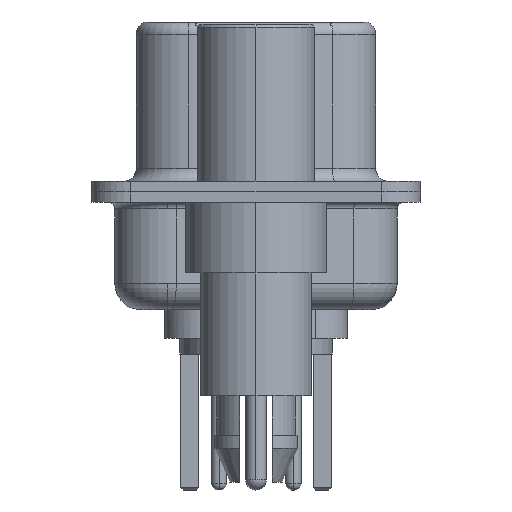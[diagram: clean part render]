
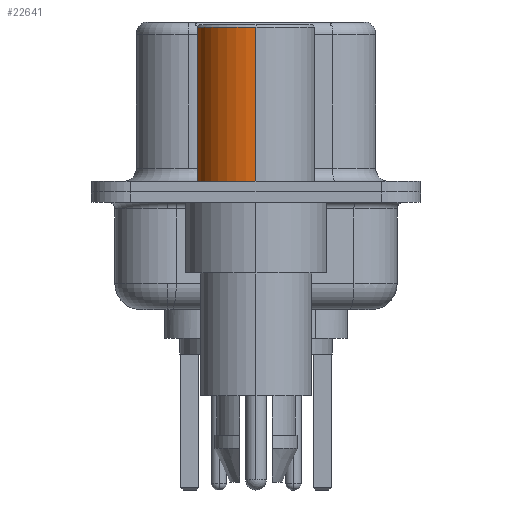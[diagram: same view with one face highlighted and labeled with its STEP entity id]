
A CAD part, left-side view. The second image highlights one B-rep face of the part: STEP entity #22641.
In plain terms, the highlighted cylindrical face has radius 2.25 mm (diameter 4.5 mm), a partial arc.
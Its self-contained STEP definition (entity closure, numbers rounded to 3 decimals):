
#1869 = CARTESIAN_POINT ( 'NONE',  ( -2.25, 0., 0.581 ) ) ;
#3920 = DIRECTION ( 'NONE',  ( 0., 0., 1. ) ) ;
#3991 = LINE ( 'NONE', #20958, #14371 ) ;
#4798 = CIRCLE ( 'NONE', #10712, 2.25 ) ;
#5557 = DIRECTION ( 'NONE',  ( 0., 0., 1. ) ) ;
#6563 = DIRECTION ( 'NONE',  ( 0., 0., 1. ) ) ;
#7270 = DIRECTION ( 'NONE',  ( 0., 0., 1. ) ) ;
#7772 = CARTESIAN_POINT ( 'NONE',  ( -2.25, 0., 0.4 ) ) ;
#7852 = CARTESIAN_POINT ( 'NONE',  ( 0., 0., 0.581 ) ) ;
#8771 = EDGE_CURVE ( 'NONE', #23547, #17788, #4798, .T. ) ;
#9093 = ORIENTED_EDGE ( 'NONE', *, *, #8771, .F. ) ;
#9204 = EDGE_LOOP ( 'NONE', ( #21386, #17923, #9093, #24444 ) ) ;
#9777 = DIRECTION ( 'NONE',  ( 1., 0., 0. ) ) ;
#10712 = AXIS2_PLACEMENT_3D ( 'NONE', #18305, #6563, #20258 ) ;
#10781 = VECTOR ( 'NONE', #19512, 1000. ) ;
#11620 = CARTESIAN_POINT ( 'NONE',  ( 2.25, 0., 6.3 ) ) ;
#11988 = EDGE_CURVE ( 'NONE', #22610, #17788, #16039, .T. ) ;
#12101 = AXIS2_PLACEMENT_3D ( 'NONE', #7852, #3920, #9777 ) ;
#13115 = EDGE_CURVE ( 'NONE', #23198, #22610, #24786, .T. ) ;
#13426 = FACE_OUTER_BOUND ( 'NONE', #9204, .T. ) ;
#14371 = VECTOR ( 'NONE', #7270, 1000. ) ;
#15485 = EDGE_CURVE ( 'NONE', #23198, #23547, #3991, .T. ) ;
#16039 = LINE ( 'NONE', #1869, #10781 ) ;
#16449 = CARTESIAN_POINT ( 'NONE',  ( -2.25, 0., 6.3 ) ) ;
#16923 = AXIS2_PLACEMENT_3D ( 'NONE', #17286, #5557, #19222 ) ;
#17286 = CARTESIAN_POINT ( 'NONE',  ( 0., 0., 0.4 ) ) ;
#17788 = VERTEX_POINT ( 'NONE', #16449 ) ;
#17923 = ORIENTED_EDGE ( 'NONE', *, *, #11988, .T. ) ;
#18305 = CARTESIAN_POINT ( 'NONE',  ( 0., 0., 6.3 ) ) ;
#19222 = DIRECTION ( 'NONE',  ( 1., 0., 0. ) ) ;
#19512 = DIRECTION ( 'NONE',  ( 0., 0., 1. ) ) ;
#20258 = DIRECTION ( 'NONE',  ( 1., 0., 0. ) ) ;
#20355 = CARTESIAN_POINT ( 'NONE',  ( 2.25, 0., 0.4 ) ) ;
#20958 = CARTESIAN_POINT ( 'NONE',  ( 2.25, 0., 0.581 ) ) ;
#21386 = ORIENTED_EDGE ( 'NONE', *, *, #13115, .T. ) ;
#22610 = VERTEX_POINT ( 'NONE', #7772 ) ;
#22641 = ADVANCED_FACE ( 'NONE', ( #13426 ), #23185, .T. ) ;
#23185 = CYLINDRICAL_SURFACE ( 'NONE', #12101, 2.25 ) ;
#23198 = VERTEX_POINT ( 'NONE', #20355 ) ;
#23547 = VERTEX_POINT ( 'NONE', #11620 ) ;
#24444 = ORIENTED_EDGE ( 'NONE', *, *, #15485, .F. ) ;
#24786 = CIRCLE ( 'NONE', #16923, 2.25 ) ;
